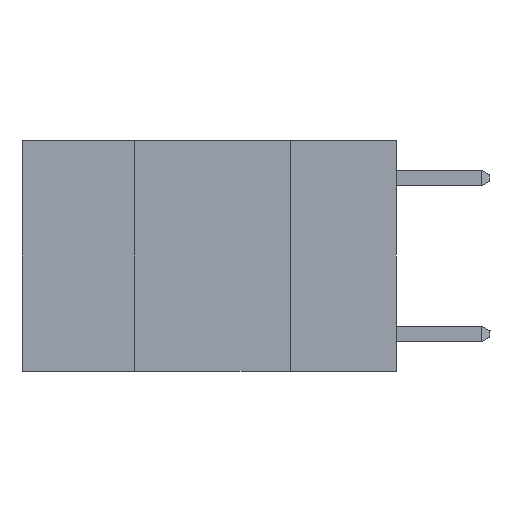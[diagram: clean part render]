
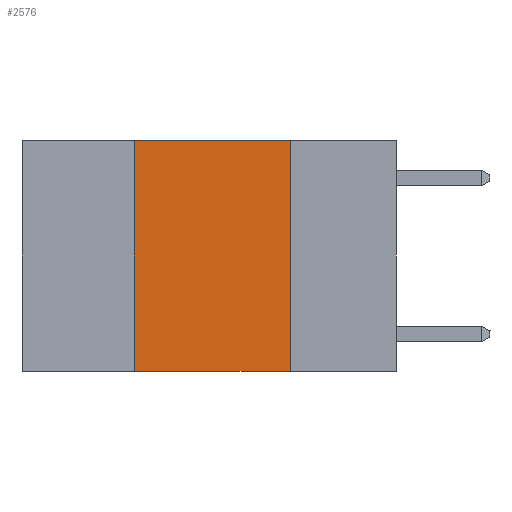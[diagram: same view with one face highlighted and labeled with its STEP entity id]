
A CAD part, left-side view. The second image highlights one B-rep face of the part: STEP entity #2576.
In plain terms, the highlighted planar face has unit normal (-1, 0, 0).
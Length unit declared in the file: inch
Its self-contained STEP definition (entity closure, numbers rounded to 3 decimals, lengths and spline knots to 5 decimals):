
#1626 = VECTOR ( 'NONE', #7909, 39.37008 ) ;
#2569 = VERTEX_POINT ( 'NONE', #24460 ) ;
#2576 = ADVANCED_FACE ( 'NONE', ( #7914 ), #17509, .F. ) ;
#3909 = LINE ( 'NONE', #12832, #28069 ) ;
#5561 = CARTESIAN_POINT ( 'NONE',  ( 0., 0.17, 0. ) ) ;
#5759 = CARTESIAN_POINT ( 'NONE',  ( 0., 0.6, 0. ) ) ;
#5984 = ORIENTED_EDGE ( 'NONE', *, *, #26604, .F. ) ;
#6317 = DIRECTION ( 'NONE',  ( 0., -1., 0. ) ) ;
#7909 = DIRECTION ( 'NONE',  ( 0., 0., -1. ) ) ;
#7914 = FACE_OUTER_BOUND ( 'NONE', #14853, .T. ) ;
#8132 = DIRECTION ( 'NONE',  ( 0., 0., -1. ) ) ;
#8503 = EDGE_CURVE ( 'NONE', #13516, #14557, #25968, .T. ) ;
#8754 = VECTOR ( 'NONE', #6317, 39.37008 ) ;
#8978 = AXIS2_PLACEMENT_3D ( 'NONE', #5759, #22233, #8132 ) ;
#9210 = DIRECTION ( 'NONE',  ( 0., -1., 0. ) ) ;
#11606 = CARTESIAN_POINT ( 'NONE',  ( 0., 0.6, -0.37 ) ) ;
#11732 = CARTESIAN_POINT ( 'NONE',  ( 0., 0.17, -0.37 ) ) ;
#12165 = CARTESIAN_POINT ( 'NONE',  ( 0., 0.17, 0. ) ) ;
#12832 = CARTESIAN_POINT ( 'NONE',  ( 0., 0.42, 0. ) ) ;
#13516 = VERTEX_POINT ( 'NONE', #23096 ) ;
#14147 = VERTEX_POINT ( 'NONE', #11732 ) ;
#14557 = VERTEX_POINT ( 'NONE', #12165 ) ;
#14853 = EDGE_LOOP ( 'NONE', ( #22032, #29416, #5984, #26417 ) ) ;
#17506 = DIRECTION ( 'NONE',  ( 0., 0., 1. ) ) ;
#17509 = PLANE ( 'NONE',  #8978 ) ;
#20356 = VECTOR ( 'NONE', #9210, 39.37008 ) ;
#20418 = CARTESIAN_POINT ( 'NONE',  ( 0., 0.6, 0. ) ) ;
#20427 = EDGE_CURVE ( 'NONE', #14557, #14147, #20443, .T. ) ;
#20443 = LINE ( 'NONE', #5561, #1626 ) ;
#21090 = LINE ( 'NONE', #11606, #20356 ) ;
#21814 = EDGE_CURVE ( 'NONE', #2569, #14147, #21090, .T. ) ;
#22032 = ORIENTED_EDGE ( 'NONE', *, *, #20427, .F. ) ;
#22233 = DIRECTION ( 'NONE',  ( 1., 0., 0. ) ) ;
#23096 = CARTESIAN_POINT ( 'NONE',  ( 0., 0.42, 0. ) ) ;
#24460 = CARTESIAN_POINT ( 'NONE',  ( 0., 0.42, -0.37 ) ) ;
#25968 = LINE ( 'NONE', #20418, #8754 ) ;
#26417 = ORIENTED_EDGE ( 'NONE', *, *, #21814, .T. ) ;
#26604 = EDGE_CURVE ( 'NONE', #2569, #13516, #3909, .T. ) ;
#28069 = VECTOR ( 'NONE', #17506, 39.37008 ) ;
#29416 = ORIENTED_EDGE ( 'NONE', *, *, #8503, .F. ) ;
